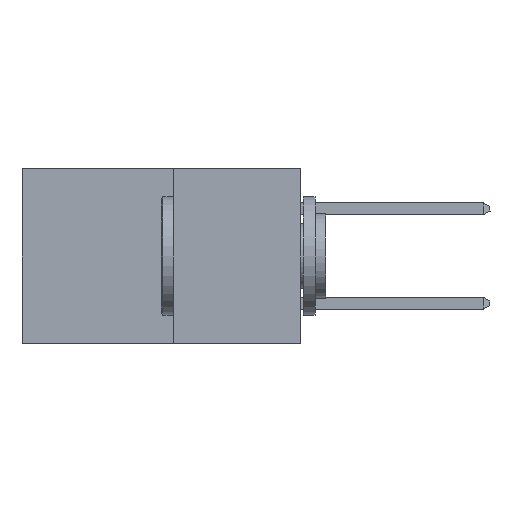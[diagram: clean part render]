
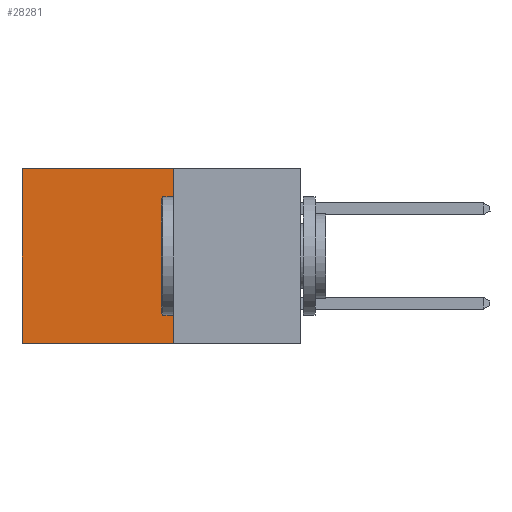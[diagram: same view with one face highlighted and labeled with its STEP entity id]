
A CAD part, left-side view. The second image highlights one B-rep face of the part: STEP entity #28281.
In plain terms, the highlighted planar face has unit normal (-1, 0, 0).
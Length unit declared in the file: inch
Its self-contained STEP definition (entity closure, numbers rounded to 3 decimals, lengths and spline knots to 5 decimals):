
#774 = CARTESIAN_POINT ( 'NONE',  ( 0.277, 0.27, -0.37 ) ) ;
#988 = ORIENTED_EDGE ( 'NONE', *, *, #4244, .F. ) ;
#1049 = CARTESIAN_POINT ( 'NONE',  ( 0.277, 0.27, -0.37 ) ) ;
#1412 = LINE ( 'NONE', #35497, #15288 ) ;
#2433 = VERTEX_POINT ( 'NONE', #29407 ) ;
#2837 = EDGE_CURVE ( 'NONE', #2433, #14951, #26270, .T. ) ;
#3847 = DIRECTION ( 'NONE',  ( 0., 0., -1. ) ) ;
#4244 = EDGE_CURVE ( 'NONE', #2433, #21846, #1412, .T. ) ;
#6929 = FACE_OUTER_BOUND ( 'NONE', #15255, .T. ) ;
#7825 = LINE ( 'NONE', #774, #29092 ) ;
#7849 = ORIENTED_EDGE ( 'NONE', *, *, #2837, .T. ) ;
#9332 = PLANE ( 'NONE',  #33763 ) ;
#11493 = VECTOR ( 'NONE', #31005, 39.37008 ) ;
#14951 = VERTEX_POINT ( 'NONE', #25742 ) ;
#15255 = EDGE_LOOP ( 'NONE', ( #21204, #29609, #988, #7849 ) ) ;
#15288 = VECTOR ( 'NONE', #34647, 39.37008 ) ;
#16337 = LINE ( 'NONE', #22201, #17193 ) ;
#17193 = VECTOR ( 'NONE', #30562, 39.37008 ) ;
#18004 = CARTESIAN_POINT ( 'NONE',  ( 0.277, 0.27, -0.37 ) ) ;
#20489 = DIRECTION ( 'NONE',  ( 1., 0., 0. ) ) ;
#21204 = ORIENTED_EDGE ( 'NONE', *, *, #25995, .T. ) ;
#21620 = VERTEX_POINT ( 'NONE', #33636 ) ;
#21846 = VERTEX_POINT ( 'NONE', #18004 ) ;
#22201 = CARTESIAN_POINT ( 'NONE',  ( 0.277, 0.59, -0.37 ) ) ;
#23987 = EDGE_CURVE ( 'NONE', #21846, #21620, #7825, .T. ) ;
#25742 = CARTESIAN_POINT ( 'NONE',  ( 0.277, 0.59, 0. ) ) ;
#25995 = EDGE_CURVE ( 'NONE', #14951, #21620, #16337, .T. ) ;
#26270 = LINE ( 'NONE', #30040, #11493 ) ;
#28281 = ADVANCED_FACE ( 'NONE', ( #6929 ), #9332, .F. ) ;
#28464 = DIRECTION ( 'NONE',  ( 0., 1., 0. ) ) ;
#29092 = VECTOR ( 'NONE', #28464, 39.37008 ) ;
#29407 = CARTESIAN_POINT ( 'NONE',  ( 0.277, 0.27, 0. ) ) ;
#29609 = ORIENTED_EDGE ( 'NONE', *, *, #23987, .F. ) ;
#30040 = CARTESIAN_POINT ( 'NONE',  ( 0.277, 0.27, 0. ) ) ;
#30562 = DIRECTION ( 'NONE',  ( 0., 0., -1. ) ) ;
#31005 = DIRECTION ( 'NONE',  ( 0., 1., 0. ) ) ;
#33636 = CARTESIAN_POINT ( 'NONE',  ( 0.277, 0.59, -0.37 ) ) ;
#33763 = AXIS2_PLACEMENT_3D ( 'NONE', #1049, #20489, #3847 ) ;
#34647 = DIRECTION ( 'NONE',  ( 0., 0., -1. ) ) ;
#35497 = CARTESIAN_POINT ( 'NONE',  ( 0.277, 0.27, -0.37 ) ) ;
